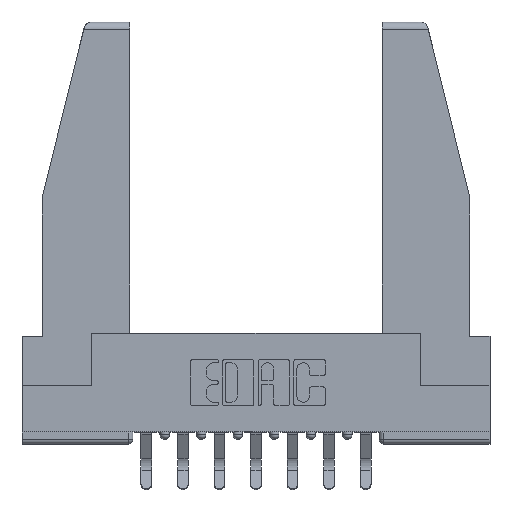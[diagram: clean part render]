
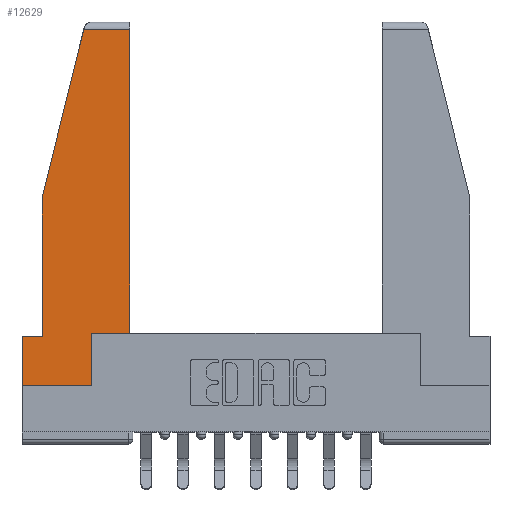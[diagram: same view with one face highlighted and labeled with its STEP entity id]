
A CAD part, top view. The second image highlights one B-rep face of the part: STEP entity #12629.
In plain terms, the highlighted planar face has unit normal (0, 0, 1).
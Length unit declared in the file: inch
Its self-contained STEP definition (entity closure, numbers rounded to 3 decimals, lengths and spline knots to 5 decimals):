
#224 = VECTOR ( 'NONE', #3291, 39.37008 ) ;
#262 = AXIS2_PLACEMENT_3D ( 'NONE', #3290, #9165, #1086 ) ;
#337 = VECTOR ( 'NONE', #11604, 39.37008 ) ;
#364 = LINE ( 'NONE', #10732, #1339 ) ;
#388 = EDGE_CURVE ( 'NONE', #6905, #1978, #6368, .T. ) ;
#588 = CARTESIAN_POINT ( 'NONE',  ( 0., 0.21, 0. ) ) ;
#711 = VERTEX_POINT ( 'NONE', #2093 ) ;
#796 = ORIENTED_EDGE ( 'NONE', *, *, #10165, .T. ) ;
#798 = CARTESIAN_POINT ( 'NONE',  ( 0., 0., 0. ) ) ;
#829 = LINE ( 'NONE', #11361, #12831 ) ;
#1086 = DIRECTION ( 'NONE',  ( 1., 0., 0. ) ) ;
#1339 = VECTOR ( 'NONE', #12723, 39.37008 ) ;
#1467 = ORIENTED_EDGE ( 'NONE', *, *, #4905, .T. ) ;
#1660 = ORIENTED_EDGE ( 'NONE', *, *, #8828, .T. ) ;
#1978 = VERTEX_POINT ( 'NONE', #10047 ) ;
#2028 = VERTEX_POINT ( 'NONE', #798 ) ;
#2093 = CARTESIAN_POINT ( 'NONE',  ( 0.461, 0.223, 0. ) ) ;
#2129 = CARTESIAN_POINT ( 'NONE',  ( 0., 1.52, 0. ) ) ;
#2192 = CARTESIAN_POINT ( 'NONE',  ( 0.271, 1.55, 0. ) ) ;
#2480 = LINE ( 'NONE', #12069, #3123 ) ;
#2500 = VERTEX_POINT ( 'NONE', #12360 ) ;
#3002 = DIRECTION ( 'NONE',  ( -1., 0., 0. ) ) ;
#3123 = VECTOR ( 'NONE', #3002, 39.37008 ) ;
#3131 = DIRECTION ( 'NONE',  ( -1., 0., 0. ) ) ;
#3242 = ORIENTED_EDGE ( 'NONE', *, *, #9163, .T. ) ;
#3290 = CARTESIAN_POINT ( 'NONE',  ( 0., 0., 0. ) ) ;
#3291 = DIRECTION ( 'NONE',  ( -0.239, -0.971, 0. ) ) ;
#4043 = CARTESIAN_POINT ( 'NONE',  ( 0.2636, 1.52, 0. ) ) ;
#4880 = EDGE_CURVE ( 'NONE', #11165, #2500, #8607, .T. ) ;
#4905 = EDGE_CURVE ( 'NONE', #11864, #9359, #2480, .T. ) ;
#5714 = VECTOR ( 'NONE', #11559, 39.37008 ) ;
#6368 = LINE ( 'NONE', #2192, #224 ) ;
#6561 = CARTESIAN_POINT ( 'NONE',  ( 0., 0., 0. ) ) ;
#6815 = ORIENTED_EDGE ( 'NONE', *, *, #11303, .T. ) ;
#6846 = CARTESIAN_POINT ( 'NONE',  ( 0.461, 1.52, 0. ) ) ;
#6905 = VERTEX_POINT ( 'NONE', #4043 ) ;
#7060 = DIRECTION ( 'NONE',  ( 0., 1., 0. ) ) ;
#7305 = LINE ( 'NONE', #6561, #5714 ) ;
#7313 = ORIENTED_EDGE ( 'NONE', *, *, #10495, .T. ) ;
#7817 = ORIENTED_EDGE ( 'NONE', *, *, #388, .T. ) ;
#8607 = LINE ( 'NONE', #12114, #12286 ) ;
#8828 = EDGE_CURVE ( 'NONE', #9359, #2028, #12121, .T. ) ;
#9163 = EDGE_CURVE ( 'NONE', #13006, #6905, #9230, .T. ) ;
#9165 = DIRECTION ( 'NONE',  ( 0., 0., 1. ) ) ;
#9230 = LINE ( 'NONE', #2129, #11947 ) ;
#9359 = VERTEX_POINT ( 'NONE', #588 ) ;
#9755 = CARTESIAN_POINT ( 'NONE',  ( 0.086, 0.21, 0. ) ) ;
#9873 = CARTESIAN_POINT ( 'NONE',  ( 0., 0.21, 0. ) ) ;
#10047 = CARTESIAN_POINT ( 'NONE',  ( 0.086, 0.8, 0. ) ) ;
#10165 = EDGE_CURVE ( 'NONE', #1978, #11864, #364, .T. ) ;
#10345 = CARTESIAN_POINT ( 'NONE',  ( 0.297, 0., 0. ) ) ;
#10359 = VECTOR ( 'NONE', #10962, 39.37008 ) ;
#10495 = EDGE_CURVE ( 'NONE', #2028, #11165, #7305, .T. ) ;
#10608 = ORIENTED_EDGE ( 'NONE', *, *, #10905, .T. ) ;
#10732 = CARTESIAN_POINT ( 'NONE',  ( 0.086, 0.8, 0. ) ) ;
#10905 = EDGE_CURVE ( 'NONE', #2500, #711, #829, .T. ) ;
#10962 = DIRECTION ( 'NONE',  ( 0., -1., 0. ) ) ;
#10968 = PLANE ( 'NONE',  #262 ) ;
#10998 = ORIENTED_EDGE ( 'NONE', *, *, #4880, .T. ) ;
#11165 = VERTEX_POINT ( 'NONE', #10345 ) ;
#11303 = EDGE_CURVE ( 'NONE', #711, #13006, #12981, .T. ) ;
#11361 = CARTESIAN_POINT ( 'NONE',  ( 0.297, 0.223, 0. ) ) ;
#11408 = FACE_OUTER_BOUND ( 'NONE', #13003, .T. ) ;
#11437 = CARTESIAN_POINT ( 'NONE',  ( 0.461, 0.223, 0. ) ) ;
#11559 = DIRECTION ( 'NONE',  ( 1., 0., 0. ) ) ;
#11604 = DIRECTION ( 'NONE',  ( 0., 1., 0. ) ) ;
#11864 = VERTEX_POINT ( 'NONE', #9755 ) ;
#11947 = VECTOR ( 'NONE', #3131, 39.37008 ) ;
#12069 = CARTESIAN_POINT ( 'NONE',  ( 0., 0.21, 0. ) ) ;
#12114 = CARTESIAN_POINT ( 'NONE',  ( 0.297, 0., 0. ) ) ;
#12121 = LINE ( 'NONE', #9873, #10359 ) ;
#12286 = VECTOR ( 'NONE', #7060, 39.37008 ) ;
#12360 = CARTESIAN_POINT ( 'NONE',  ( 0.297, 0.223, 0. ) ) ;
#12369 = DIRECTION ( 'NONE',  ( 1., 0., 0. ) ) ;
#12629 = ADVANCED_FACE ( 'NONE', ( #11408 ), #10968, .T. ) ;
#12723 = DIRECTION ( 'NONE',  ( 0., -1., 0. ) ) ;
#12831 = VECTOR ( 'NONE', #12369, 39.37008 ) ;
#12981 = LINE ( 'NONE', #11437, #337 ) ;
#13003 = EDGE_LOOP ( 'NONE', ( #6815, #3242, #7817, #796, #1467, #1660, #7313, #10998, #10608 ) ) ;
#13006 = VERTEX_POINT ( 'NONE', #6846 ) ;
